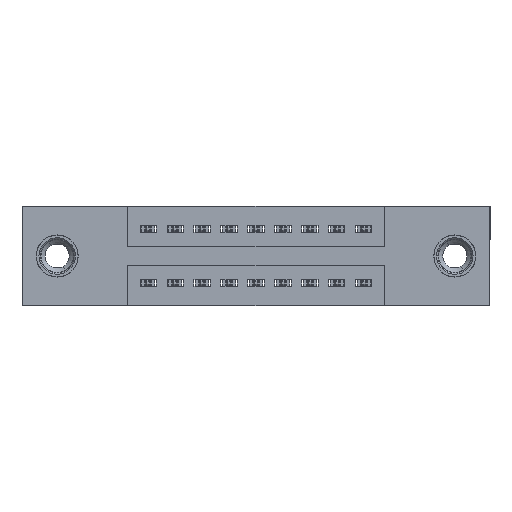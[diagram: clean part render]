
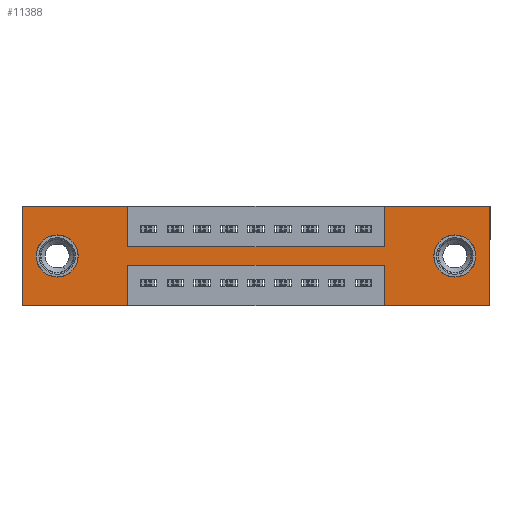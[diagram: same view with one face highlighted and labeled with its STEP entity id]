
A CAD part, front view. The second image highlights one B-rep face of the part: STEP entity #11388.
In plain terms, the highlighted planar face has unit normal (0, -1, 0).
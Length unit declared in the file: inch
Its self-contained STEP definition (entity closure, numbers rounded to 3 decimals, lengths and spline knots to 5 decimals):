
#95 = CIRCLE ( 'NONE', #13210, 0.078 ) ;
#161 = CARTESIAN_POINT ( 'NONE',  ( 0., 0., -0.37 ) ) ;
#513 = VECTOR ( 'NONE', #9436, 39.37008 ) ;
#551 = CARTESIAN_POINT ( 'NONE',  ( 1.735, 0., -0.37 ) ) ;
#599 = ORIENTED_EDGE ( 'NONE', *, *, #11072, .T. ) ;
#614 = DIRECTION ( 'NONE',  ( 0., 0., -1. ) ) ;
#732 = EDGE_CURVE ( 'NONE', #10209, #3351, #6415, .T. ) ;
#1148 = VECTOR ( 'NONE', #15509, 39.37008 ) ;
#1506 = DIRECTION ( 'NONE',  ( -1., 0., 0. ) ) ;
#1568 = DIRECTION ( 'NONE',  ( 0., 0., -1. ) ) ;
#1670 = CARTESIAN_POINT ( 'NONE',  ( 0., 0., -0.37 ) ) ;
#1990 = DIRECTION ( 'NONE',  ( 0., 0., 1. ) ) ;
#2046 = EDGE_CURVE ( 'NONE', #4594, #4782, #2526, .T. ) ;
#2266 = ORIENTED_EDGE ( 'NONE', *, *, #2967, .T. ) ;
#2270 = CARTESIAN_POINT ( 'NONE',  ( 0.13, 0., -0.185 ) ) ;
#2297 = CARTESIAN_POINT ( 'NONE',  ( 1.3425, 0., -0.15 ) ) ;
#2326 = ORIENTED_EDGE ( 'NONE', *, *, #11156, .T. ) ;
#2342 = VERTEX_POINT ( 'NONE', #15777 ) ;
#2349 = AXIS2_PLACEMENT_3D ( 'NONE', #3510, #12301, #4835 ) ;
#2526 = LINE ( 'NONE', #7204, #8997 ) ;
#2537 = DIRECTION ( 'NONE',  ( 0., 1., 0. ) ) ;
#2546 = VECTOR ( 'NONE', #13290, 39.37008 ) ;
#2568 = AXIS2_PLACEMENT_3D ( 'NONE', #10227, #2537, #11426 ) ;
#2967 = EDGE_CURVE ( 'NONE', #2995, #7293, #7589, .T. ) ;
#2995 = VERTEX_POINT ( 'NONE', #6469 ) ;
#3284 = CARTESIAN_POINT ( 'NONE',  ( 0.3925, 0., 0. ) ) ;
#3305 = LINE ( 'NONE', #6089, #12925 ) ;
#3351 = VERTEX_POINT ( 'NONE', #551 ) ;
#3493 = EDGE_CURVE ( 'NONE', #4563, #13678, #3305, .T. ) ;
#3505 = EDGE_CURVE ( 'NONE', #7293, #2995, #95, .T. ) ;
#3510 = CARTESIAN_POINT ( 'NONE',  ( 1.605, 0., -0.185 ) ) ;
#3625 = DIRECTION ( 'NONE',  ( 0., 0., 1. ) ) ;
#3828 = VERTEX_POINT ( 'NONE', #6787 ) ;
#4020 = ORIENTED_EDGE ( 'NONE', *, *, #14900, .F. ) ;
#4033 = EDGE_CURVE ( 'NONE', #7531, #10209, #10105, .T. ) ;
#4103 = DIRECTION ( 'NONE',  ( -1., 0., 0. ) ) ;
#4403 = EDGE_CURVE ( 'NONE', #13678, #3828, #14019, .T. ) ;
#4563 = VERTEX_POINT ( 'NONE', #9707 ) ;
#4594 = VERTEX_POINT ( 'NONE', #4645 ) ;
#4645 = CARTESIAN_POINT ( 'NONE',  ( 0.3925, 0., -0.15 ) ) ;
#4782 = VERTEX_POINT ( 'NONE', #2297 ) ;
#4835 = DIRECTION ( 'NONE',  ( 0., 0., -1. ) ) ;
#4928 = CARTESIAN_POINT ( 'NONE',  ( 0., 0., 0. ) ) ;
#4970 = CARTESIAN_POINT ( 'NONE',  ( 0.13, 0., -0.107 ) ) ;
#5002 = EDGE_LOOP ( 'NONE', ( #14517, #2266 ) ) ;
#5723 = FACE_OUTER_BOUND ( 'NONE', #9488, .T. ) ;
#5807 = CARTESIAN_POINT ( 'NONE',  ( 0.3925, 0., -0.37 ) ) ;
#5950 = DIRECTION ( 'NONE',  ( 1., 0., 0. ) ) ;
#5961 = EDGE_CURVE ( 'NONE', #3828, #14313, #8118, .T. ) ;
#6089 = CARTESIAN_POINT ( 'NONE',  ( 0.3925, 0., -0.37 ) ) ;
#6128 = FACE_BOUND ( 'NONE', #10779, .T. ) ;
#6144 = DIRECTION ( 'NONE',  ( 0., 0., -1. ) ) ;
#6243 = VECTOR ( 'NONE', #12108, 39.37008 ) ;
#6290 = VERTEX_POINT ( 'NONE', #10330 ) ;
#6359 = VERTEX_POINT ( 'NONE', #12829 ) ;
#6415 = LINE ( 'NONE', #13195, #2546 ) ;
#6469 = CARTESIAN_POINT ( 'NONE',  ( 0.13, 0., -0.263 ) ) ;
#6549 = ORIENTED_EDGE ( 'NONE', *, *, #2046, .F. ) ;
#6657 = LINE ( 'NONE', #15167, #10015 ) ;
#6787 = CARTESIAN_POINT ( 'NONE',  ( 0., 0., -0.37 ) ) ;
#6979 = LINE ( 'NONE', #12735, #10331 ) ;
#7204 = CARTESIAN_POINT ( 'NONE',  ( 0.3925, 0., -0.15 ) ) ;
#7293 = VERTEX_POINT ( 'NONE', #4970 ) ;
#7531 = VERTEX_POINT ( 'NONE', #15188 ) ;
#7589 = CIRCLE ( 'NONE', #2568, 0.078 ) ;
#7775 = VERTEX_POINT ( 'NONE', #8426 ) ;
#8118 = LINE ( 'NONE', #8266, #1148 ) ;
#8133 = EDGE_CURVE ( 'NONE', #14313, #6290, #8239, .T. ) ;
#8239 = LINE ( 'NONE', #8674, #14302 ) ;
#8266 = CARTESIAN_POINT ( 'NONE',  ( 0., 0., 0. ) ) ;
#8426 = CARTESIAN_POINT ( 'NONE',  ( 1.605, 0., -0.263 ) ) ;
#8475 = DIRECTION ( 'NONE',  ( 0., 1., 0. ) ) ;
#8674 = CARTESIAN_POINT ( 'NONE',  ( 0., 0., 0. ) ) ;
#8962 = CIRCLE ( 'NONE', #2349, 0.078 ) ;
#8997 = VECTOR ( 'NONE', #5950, 39.37008 ) ;
#9146 = DIRECTION ( 'NONE',  ( 0., 0., 1. ) ) ;
#9165 = CARTESIAN_POINT ( 'NONE',  ( 1.735, 0., 0. ) ) ;
#9283 = CARTESIAN_POINT ( 'NONE',  ( 0.3925, 0., -0.22 ) ) ;
#9336 = DIRECTION ( 'NONE',  ( 0., -1., 0. ) ) ;
#9436 = DIRECTION ( 'NONE',  ( -1., 0., 0. ) ) ;
#9488 = EDGE_LOOP ( 'NONE', ( #11120, #9708, #4020, #9852, #12758, #13221, #12901, #6549, #11150, #10317, #12587, #13396 ) ) ;
#9596 = AXIS2_PLACEMENT_3D ( 'NONE', #15707, #8475, #614 ) ;
#9648 = LINE ( 'NONE', #3284, #6243 ) ;
#9707 = CARTESIAN_POINT ( 'NONE',  ( 0.3925, 0., -0.22 ) ) ;
#9708 = ORIENTED_EDGE ( 'NONE', *, *, #13227, .F. ) ;
#9724 = VECTOR ( 'NONE', #10039, 39.37008 ) ;
#9749 = CARTESIAN_POINT ( 'NONE',  ( 1.3425, 0., -0.37 ) ) ;
#9852 = ORIENTED_EDGE ( 'NONE', *, *, #13179, .F. ) ;
#10015 = VECTOR ( 'NONE', #4103, 39.37008 ) ;
#10039 = DIRECTION ( 'NONE',  ( 1., 0., 0. ) ) ;
#10105 = LINE ( 'NONE', #4928, #9724 ) ;
#10209 = VERTEX_POINT ( 'NONE', #9165 ) ;
#10227 = CARTESIAN_POINT ( 'NONE',  ( 0.13, 0., -0.185 ) ) ;
#10317 = ORIENTED_EDGE ( 'NONE', *, *, #8133, .F. ) ;
#10330 = CARTESIAN_POINT ( 'NONE',  ( 0.3925, 0., 0. ) ) ;
#10331 = VECTOR ( 'NONE', #9146, 39.37008 ) ;
#10423 = PLANE ( 'NONE',  #10630 ) ;
#10630 = AXIS2_PLACEMENT_3D ( 'NONE', #161, #9336, #1568 ) ;
#10779 = EDGE_LOOP ( 'NONE', ( #2326, #599 ) ) ;
#10832 = EDGE_CURVE ( 'NONE', #4782, #7531, #6979, .T. ) ;
#11072 = EDGE_CURVE ( 'NONE', #7775, #2342, #16101, .T. ) ;
#11120 = ORIENTED_EDGE ( 'NONE', *, *, #3493, .F. ) ;
#11150 = ORIENTED_EDGE ( 'NONE', *, *, #12721, .F. ) ;
#11156 = EDGE_CURVE ( 'NONE', #2342, #7775, #8962, .T. ) ;
#11207 = DIRECTION ( 'NONE',  ( 0., 1., 0. ) ) ;
#11388 = ADVANCED_FACE ( 'NONE', ( #6128, #12359, #5723 ), #10423, .T. ) ;
#11426 = DIRECTION ( 'NONE',  ( 0., 0., 1. ) ) ;
#11457 = LINE ( 'NONE', #9749, #14619 ) ;
#12084 = LINE ( 'NONE', #9283, #15621 ) ;
#12108 = DIRECTION ( 'NONE',  ( 0., 0., -1. ) ) ;
#12301 = DIRECTION ( 'NONE',  ( 0., 1., 0. ) ) ;
#12359 = FACE_BOUND ( 'NONE', #5002, .T. ) ;
#12587 = ORIENTED_EDGE ( 'NONE', *, *, #5961, .F. ) ;
#12721 = EDGE_CURVE ( 'NONE', #6290, #4594, #9648, .T. ) ;
#12735 = CARTESIAN_POINT ( 'NONE',  ( 1.3425, 0., 0. ) ) ;
#12758 = ORIENTED_EDGE ( 'NONE', *, *, #732, .F. ) ;
#12829 = CARTESIAN_POINT ( 'NONE',  ( 1.3425, 0., -0.37 ) ) ;
#12901 = ORIENTED_EDGE ( 'NONE', *, *, #10832, .F. ) ;
#12925 = VECTOR ( 'NONE', #6144, 39.37008 ) ;
#13179 = EDGE_CURVE ( 'NONE', #3351, #6359, #6657, .T. ) ;
#13195 = CARTESIAN_POINT ( 'NONE',  ( 1.735, 0., 0. ) ) ;
#13210 = AXIS2_PLACEMENT_3D ( 'NONE', #2270, #11207, #3625 ) ;
#13221 = ORIENTED_EDGE ( 'NONE', *, *, #4033, .F. ) ;
#13227 = EDGE_CURVE ( 'NONE', #14241, #4563, #12084, .T. ) ;
#13290 = DIRECTION ( 'NONE',  ( 0., 0., -1. ) ) ;
#13318 = CARTESIAN_POINT ( 'NONE',  ( 0., 0., 0. ) ) ;
#13396 = ORIENTED_EDGE ( 'NONE', *, *, #4403, .F. ) ;
#13678 = VERTEX_POINT ( 'NONE', #5807 ) ;
#14019 = LINE ( 'NONE', #1670, #513 ) ;
#14241 = VERTEX_POINT ( 'NONE', #14372 ) ;
#14302 = VECTOR ( 'NONE', #15884, 39.37008 ) ;
#14313 = VERTEX_POINT ( 'NONE', #13318 ) ;
#14372 = CARTESIAN_POINT ( 'NONE',  ( 1.3425, 0., -0.22 ) ) ;
#14517 = ORIENTED_EDGE ( 'NONE', *, *, #3505, .T. ) ;
#14619 = VECTOR ( 'NONE', #1990, 39.37008 ) ;
#14900 = EDGE_CURVE ( 'NONE', #6359, #14241, #11457, .T. ) ;
#15167 = CARTESIAN_POINT ( 'NONE',  ( 0., 0., -0.37 ) ) ;
#15188 = CARTESIAN_POINT ( 'NONE',  ( 1.3425, 0., 0. ) ) ;
#15509 = DIRECTION ( 'NONE',  ( 0., 0., 1. ) ) ;
#15621 = VECTOR ( 'NONE', #1506, 39.37008 ) ;
#15707 = CARTESIAN_POINT ( 'NONE',  ( 1.605, 0., -0.185 ) ) ;
#15777 = CARTESIAN_POINT ( 'NONE',  ( 1.605, 0., -0.107 ) ) ;
#15884 = DIRECTION ( 'NONE',  ( 1., 0., 0. ) ) ;
#16101 = CIRCLE ( 'NONE', #9596, 0.078 ) ;
